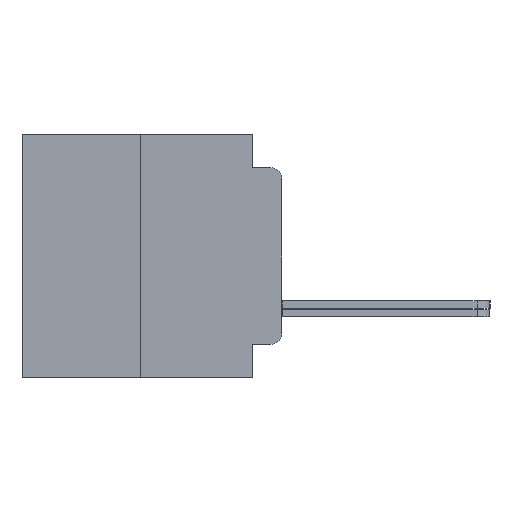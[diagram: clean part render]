
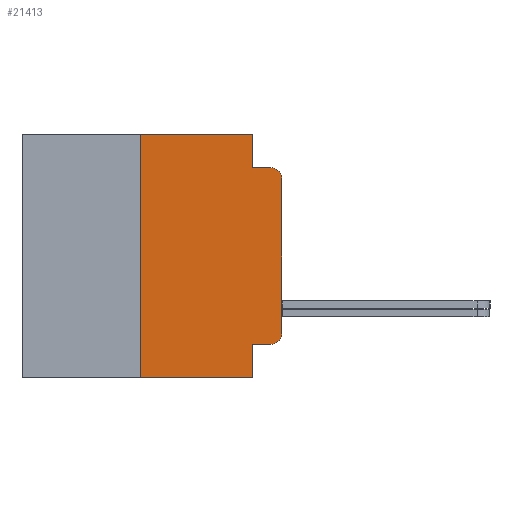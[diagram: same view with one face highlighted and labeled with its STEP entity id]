
A CAD part, left-side view. The second image highlights one B-rep face of the part: STEP entity #21413.
In plain terms, the highlighted planar face has unit normal (-1, 0, 0).
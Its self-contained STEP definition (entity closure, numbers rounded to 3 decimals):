
#12 = ORIENTED_EDGE ( 'NONE', *, *, #3591, .F. ) ;
#17 = ORIENTED_EDGE ( 'NONE', *, *, #3741, .F. ) ;
#1076 = VECTOR ( 'NONE', #24796, 1000. ) ;
#1344 = CARTESIAN_POINT ( 'NONE',  ( -75.603, 1.295, -5.486 ) ) ;
#1549 = EDGE_CURVE ( 'NONE', #8025, #13050, #22862, .T. ) ;
#2046 = VECTOR ( 'NONE', #16218, 1000. ) ;
#2434 = AXIS2_PLACEMENT_3D ( 'NONE', #18457, #16337, #18552 ) ;
#2671 = VERTEX_POINT ( 'NONE', #1344 ) ;
#3087 = AXIS2_PLACEMENT_3D ( 'NONE', #17242, #4289, #6614 ) ;
#3529 = EDGE_CURVE ( 'NONE', #20734, #13676, #20068, .T. ) ;
#3591 = EDGE_CURVE ( 'NONE', #19241, #20734, #4699, .T. ) ;
#3741 = EDGE_CURVE ( 'NONE', #25782, #2671, #6037, .T. ) ;
#3880 = VERTEX_POINT ( 'NONE', #25952 ) ;
#4289 = DIRECTION ( 'NONE',  ( -1., 0., 0. ) ) ;
#4699 = LINE ( 'NONE', #27187, #1076 ) ;
#5145 = VECTOR ( 'NONE', #15983, 1000. ) ;
#6037 = LINE ( 'NONE', #15922, #2046 ) ;
#6351 = CARTESIAN_POINT ( 'NONE',  ( -75.603, 1.295, -3.975 ) ) ;
#6416 = CARTESIAN_POINT ( 'NONE',  ( -75.603, 11.684, 5.486 ) ) ;
#6614 = DIRECTION ( 'NONE',  ( 0., 0., -1. ) ) ;
#7309 = CARTESIAN_POINT ( 'NONE',  ( -75.603, 0.508, -3.467 ) ) ;
#8025 = VERTEX_POINT ( 'NONE', #17093 ) ;
#8796 = VERTEX_POINT ( 'NONE', #21733 ) ;
#8997 = CIRCLE ( 'NONE', #10792, 0.508 ) ;
#9189 = LINE ( 'NONE', #24268, #24229 ) ;
#9652 = DIRECTION ( 'NONE',  ( 0., 0., -1. ) ) ;
#10792 = AXIS2_PLACEMENT_3D ( 'NONE', #7309, #22249, #24392 ) ;
#11336 = VECTOR ( 'NONE', #25715, 1000. ) ;
#11533 = EDGE_CURVE ( 'NONE', #19241, #2671, #21352, .T. ) ;
#12021 = FACE_OUTER_BOUND ( 'NONE', #20823, .T. ) ;
#13050 = VERTEX_POINT ( 'NONE', #14217 ) ;
#13676 = VERTEX_POINT ( 'NONE', #14655 ) ;
#13748 = ORIENTED_EDGE ( 'NONE', *, *, #11533, .T. ) ;
#14047 = CARTESIAN_POINT ( 'NONE',  ( -75.603, 1.295, 0. ) ) ;
#14217 = CARTESIAN_POINT ( 'NONE',  ( -75.603, 0., 3.467 ) ) ;
#14655 = CARTESIAN_POINT ( 'NONE',  ( -75.603, 1.295, 5.486 ) ) ;
#15044 = EDGE_CURVE ( 'NONE', #15500, #3880, #9189, .T. ) ;
#15075 = ORIENTED_EDGE ( 'NONE', *, *, #18157, .T. ) ;
#15382 = LINE ( 'NONE', #14047, #15697 ) ;
#15500 = VERTEX_POINT ( 'NONE', #17138 ) ;
#15697 = VECTOR ( 'NONE', #9652, 1000. ) ;
#15922 = CARTESIAN_POINT ( 'NONE',  ( -75.603, 1.295, 0. ) ) ;
#15983 = DIRECTION ( 'NONE',  ( 0., 0., 1. ) ) ;
#16218 = DIRECTION ( 'NONE',  ( 0., 0., -1. ) ) ;
#16276 = CARTESIAN_POINT ( 'NONE',  ( -75.603, 6.35, 5.486 ) ) ;
#16337 = DIRECTION ( 'NONE',  ( 1., 0., 0. ) ) ;
#16572 = DIRECTION ( 'NONE',  ( 0., -1., 0. ) ) ;
#16752 = ORIENTED_EDGE ( 'NONE', *, *, #15044, .F. ) ;
#17093 = CARTESIAN_POINT ( 'NONE',  ( -75.603, 0., -3.467 ) ) ;
#17138 = CARTESIAN_POINT ( 'NONE',  ( -75.603, 1.295, 3.975 ) ) ;
#17242 = CARTESIAN_POINT ( 'NONE',  ( -75.603, 0.508, 3.467 ) ) ;
#18157 = EDGE_CURVE ( 'NONE', #13050, #3880, #21582, .T. ) ;
#18296 = VECTOR ( 'NONE', #16572, 1000. ) ;
#18376 = VECTOR ( 'NONE', #21816, 1000. ) ;
#18457 = CARTESIAN_POINT ( 'NONE',  ( -75.603, 11.684, 5.486 ) ) ;
#18552 = DIRECTION ( 'NONE',  ( 0., 0., -1. ) ) ;
#18965 = LINE ( 'NONE', #24771, #18296 ) ;
#19241 = VERTEX_POINT ( 'NONE', #24867 ) ;
#20068 = LINE ( 'NONE', #6416, #18376 ) ;
#20106 = ORIENTED_EDGE ( 'NONE', *, *, #3529, .F. ) ;
#20613 = PLANE ( 'NONE',  #2434 ) ;
#20734 = VERTEX_POINT ( 'NONE', #16276 ) ;
#20823 = EDGE_LOOP ( 'NONE', ( #24365, #25215, #21660, #15075, #16752, #25563, #20106, #12, #13748, #17 ) ) ;
#21352 = LINE ( 'NONE', #21418, #11336 ) ;
#21413 = ADVANCED_FACE ( 'NONE', ( #12021 ), #20613, .F. ) ;
#21418 = CARTESIAN_POINT ( 'NONE',  ( -75.603, 11.684, -5.486 ) ) ;
#21582 = CIRCLE ( 'NONE', #3087, 0.508 ) ;
#21660 = ORIENTED_EDGE ( 'NONE', *, *, #1549, .T. ) ;
#21733 = CARTESIAN_POINT ( 'NONE',  ( -75.603, 0.508, -3.975 ) ) ;
#21816 = DIRECTION ( 'NONE',  ( 0., -1., 0. ) ) ;
#22249 = DIRECTION ( 'NONE',  ( -1., 0., 0. ) ) ;
#22862 = LINE ( 'NONE', #24849, #5145 ) ;
#23674 = EDGE_CURVE ( 'NONE', #25782, #8796, #18965, .T. ) ;
#24229 = VECTOR ( 'NONE', #24553, 1000. ) ;
#24268 = CARTESIAN_POINT ( 'NONE',  ( -75.603, 1.295, 3.975 ) ) ;
#24365 = ORIENTED_EDGE ( 'NONE', *, *, #23674, .T. ) ;
#24392 = DIRECTION ( 'NONE',  ( 0., 0., -1. ) ) ;
#24553 = DIRECTION ( 'NONE',  ( 0., -1., 0. ) ) ;
#24771 = CARTESIAN_POINT ( 'NONE',  ( -75.603, 1.295, -3.975 ) ) ;
#24796 = DIRECTION ( 'NONE',  ( 0., 0., 1. ) ) ;
#24849 = CARTESIAN_POINT ( 'NONE',  ( -75.603, 0., 5.486 ) ) ;
#24867 = CARTESIAN_POINT ( 'NONE',  ( -75.603, 6.35, -5.486 ) ) ;
#25215 = ORIENTED_EDGE ( 'NONE', *, *, #27490, .T. ) ;
#25563 = ORIENTED_EDGE ( 'NONE', *, *, #26945, .F. ) ;
#25715 = DIRECTION ( 'NONE',  ( 0., -1., 0. ) ) ;
#25782 = VERTEX_POINT ( 'NONE', #6351 ) ;
#25952 = CARTESIAN_POINT ( 'NONE',  ( -75.603, 0.508, 3.975 ) ) ;
#26945 = EDGE_CURVE ( 'NONE', #13676, #15500, #15382, .T. ) ;
#27187 = CARTESIAN_POINT ( 'NONE',  ( -75.603, 6.35, -5.486 ) ) ;
#27490 = EDGE_CURVE ( 'NONE', #8796, #8025, #8997, .T. ) ;
